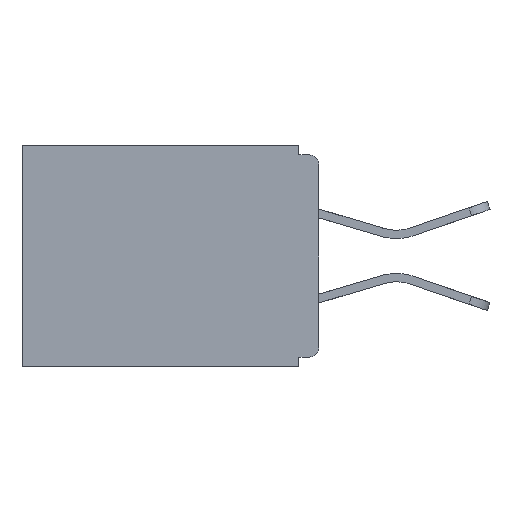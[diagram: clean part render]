
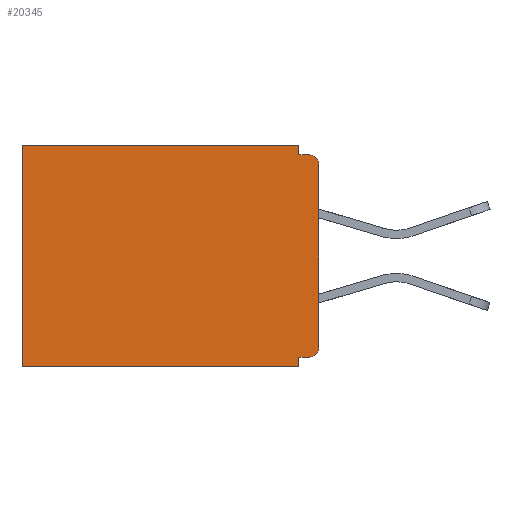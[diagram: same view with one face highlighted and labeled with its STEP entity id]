
A CAD part, left-side view. The second image highlights one B-rep face of the part: STEP entity #20345.
In plain terms, the highlighted planar face has unit normal (-1, 0, 0).
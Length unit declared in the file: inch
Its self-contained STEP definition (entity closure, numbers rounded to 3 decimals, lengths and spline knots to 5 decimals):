
#115 = VECTOR ( 'NONE', #6562, 39.37008 ) ;
#532 = VERTEX_POINT ( 'NONE', #5868 ) ;
#826 = VERTEX_POINT ( 'NONE', #20022 ) ;
#1273 = CARTESIAN_POINT ( 'NONE',  ( 0.298, 0., 0. ) ) ;
#1287 = EDGE_CURVE ( 'NONE', #20694, #4295, #24238, .T. ) ;
#1877 = ORIENTED_EDGE ( 'NONE', *, *, #5979, .T. ) ;
#2176 = EDGE_CURVE ( 'NONE', #27972, #4295, #20414, .T. ) ;
#2852 = EDGE_LOOP ( 'NONE', ( #2869, #5513, #13488, #1877, #16066, #27182, #10707, #14678, #8996, #8497 ) ) ;
#2869 = ORIENTED_EDGE ( 'NONE', *, *, #2894, .T. ) ;
#2894 = EDGE_CURVE ( 'NONE', #532, #15465, #12853, .T. ) ;
#3060 = VERTEX_POINT ( 'NONE', #17722 ) ;
#3310 = PLANE ( 'NONE',  #24499 ) ;
#3390 = DIRECTION ( 'NONE',  ( 0., 0., -1. ) ) ;
#4295 = VERTEX_POINT ( 'NONE', #23837 ) ;
#4784 = LINE ( 'NONE', #7693, #10623 ) ;
#5504 = VECTOR ( 'NONE', #12860, 39.37008 ) ;
#5513 = ORIENTED_EDGE ( 'NONE', *, *, #23262, .F. ) ;
#5743 = DIRECTION ( 'NONE',  ( 0., 0., -1. ) ) ;
#5853 = CARTESIAN_POINT ( 'NONE',  ( 0.298, 0.015, -0.03 ) ) ;
#5868 = CARTESIAN_POINT ( 'NONE',  ( 0.298, 0., -0.03 ) ) ;
#5979 = EDGE_CURVE ( 'NONE', #6720, #27972, #4784, .T. ) ;
#6266 = LINE ( 'NONE', #1273, #24158 ) ;
#6495 = CARTESIAN_POINT ( 'NONE',  ( 0.298, 0.46, 0. ) ) ;
#6562 = DIRECTION ( 'NONE',  ( 0., 0., -1. ) ) ;
#6720 = VERTEX_POINT ( 'NONE', #21689 ) ;
#7519 = LINE ( 'NONE', #17355, #18241 ) ;
#7651 = CARTESIAN_POINT ( 'NONE',  ( 0.298, 0.015, -0.313 ) ) ;
#7693 = CARTESIAN_POINT ( 'NONE',  ( 0.298, 0., 0. ) ) ;
#8198 = DIRECTION ( 'NONE',  ( 0., 1., 0. ) ) ;
#8497 = ORIENTED_EDGE ( 'NONE', *, *, #27061, .F. ) ;
#8796 = LINE ( 'NONE', #28102, #10907 ) ;
#8996 = ORIENTED_EDGE ( 'NONE', *, *, #13329, .T. ) ;
#10623 = VECTOR ( 'NONE', #18884, 39.37008 ) ;
#10707 = ORIENTED_EDGE ( 'NONE', *, *, #13664, .F. ) ;
#10907 = VECTOR ( 'NONE', #25870, 39.37008 ) ;
#12077 = DIRECTION ( 'NONE',  ( 0., 0., -1. ) ) ;
#12126 = EDGE_CURVE ( 'NONE', #6720, #21112, #23126, .T. ) ;
#12410 = DIRECTION ( 'NONE',  ( -1., 0., 0. ) ) ;
#12853 = CIRCLE ( 'NONE', #26058, 0.015 ) ;
#12860 = DIRECTION ( 'NONE',  ( 0., 0., -1. ) ) ;
#13048 = CARTESIAN_POINT ( 'NONE',  ( 0.298, 0.031, -0.343 ) ) ;
#13329 = EDGE_CURVE ( 'NONE', #3060, #826, #23783, .T. ) ;
#13488 = ORIENTED_EDGE ( 'NONE', *, *, #12126, .F. ) ;
#13664 = EDGE_CURVE ( 'NONE', #26663, #20694, #25463, .T. ) ;
#14333 = EDGE_CURVE ( 'NONE', #3060, #26663, #7519, .T. ) ;
#14374 = CARTESIAN_POINT ( 'NONE',  ( 0.298, 0.031, -0.343 ) ) ;
#14678 = ORIENTED_EDGE ( 'NONE', *, *, #14333, .F. ) ;
#15229 = VECTOR ( 'NONE', #3390, 39.37008 ) ;
#15465 = VERTEX_POINT ( 'NONE', #22871 ) ;
#16066 = ORIENTED_EDGE ( 'NONE', *, *, #2176, .T. ) ;
#16623 = CARTESIAN_POINT ( 'NONE',  ( 0.298, 0., 0. ) ) ;
#17355 = CARTESIAN_POINT ( 'NONE',  ( 0.298, 0., -0.328 ) ) ;
#17371 = CARTESIAN_POINT ( 'NONE',  ( 0.298, 0.031, -0.343 ) ) ;
#17722 = CARTESIAN_POINT ( 'NONE',  ( 0.298, 0.015, -0.328 ) ) ;
#18241 = VECTOR ( 'NONE', #25795, 39.37008 ) ;
#18884 = DIRECTION ( 'NONE',  ( 0., 1., 0. ) ) ;
#19184 = CARTESIAN_POINT ( 'NONE',  ( 0.298, 0., -0.343 ) ) ;
#19769 = CARTESIAN_POINT ( 'NONE',  ( 0.298, 0.46, 0. ) ) ;
#20022 = CARTESIAN_POINT ( 'NONE',  ( 0.298, 0., -0.313 ) ) ;
#20345 = ADVANCED_FACE ( 'NONE', ( #27929 ), #3310, .F. ) ;
#20414 = LINE ( 'NONE', #19769, #115 ) ;
#20475 = VECTOR ( 'NONE', #8198, 39.37008 ) ;
#20694 = VERTEX_POINT ( 'NONE', #17371 ) ;
#20850 = DIRECTION ( 'NONE',  ( -1., 0., 0. ) ) ;
#21112 = VERTEX_POINT ( 'NONE', #23498 ) ;
#21689 = CARTESIAN_POINT ( 'NONE',  ( 0.298, 0.031, 0. ) ) ;
#22871 = CARTESIAN_POINT ( 'NONE',  ( 0.298, 0.015, -0.015 ) ) ;
#23018 = DIRECTION ( 'NONE',  ( 0., 0., -1. ) ) ;
#23053 = AXIS2_PLACEMENT_3D ( 'NONE', #7651, #20850, #5743 ) ;
#23126 = LINE ( 'NONE', #14374, #15229 ) ;
#23262 = EDGE_CURVE ( 'NONE', #21112, #15465, #8796, .T. ) ;
#23498 = CARTESIAN_POINT ( 'NONE',  ( 0.298, 0.031, -0.015 ) ) ;
#23783 = CIRCLE ( 'NONE', #23053, 0.015 ) ;
#23837 = CARTESIAN_POINT ( 'NONE',  ( 0.298, 0.46, -0.343 ) ) ;
#24158 = VECTOR ( 'NONE', #23018, 39.37008 ) ;
#24238 = LINE ( 'NONE', #19184, #20475 ) ;
#24499 = AXIS2_PLACEMENT_3D ( 'NONE', #16623, #27374, #12077 ) ;
#25463 = LINE ( 'NONE', #13048, #5504 ) ;
#25795 = DIRECTION ( 'NONE',  ( 0., 1., 0. ) ) ;
#25870 = DIRECTION ( 'NONE',  ( 0., -1., 0. ) ) ;
#26058 = AXIS2_PLACEMENT_3D ( 'NONE', #5853, #12410, #27516 ) ;
#26320 = CARTESIAN_POINT ( 'NONE',  ( 0.298, 0.031, -0.328 ) ) ;
#26663 = VERTEX_POINT ( 'NONE', #26320 ) ;
#27061 = EDGE_CURVE ( 'NONE', #532, #826, #6266, .T. ) ;
#27182 = ORIENTED_EDGE ( 'NONE', *, *, #1287, .F. ) ;
#27374 = DIRECTION ( 'NONE',  ( 1., 0., 0. ) ) ;
#27516 = DIRECTION ( 'NONE',  ( 0., 0., -1. ) ) ;
#27929 = FACE_OUTER_BOUND ( 'NONE', #2852, .T. ) ;
#27972 = VERTEX_POINT ( 'NONE', #6495 ) ;
#28102 = CARTESIAN_POINT ( 'NONE',  ( 0.298, 0., -0.015 ) ) ;
